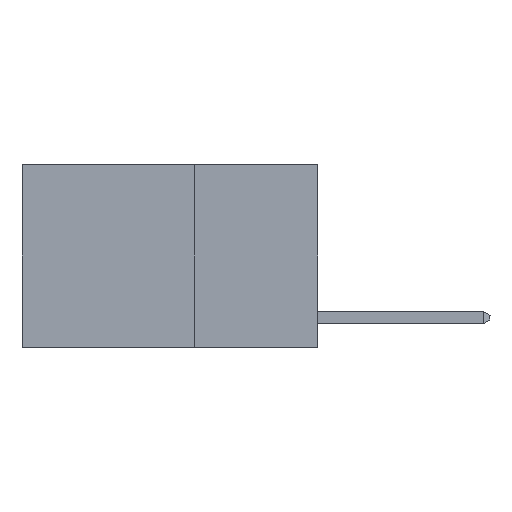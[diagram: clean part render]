
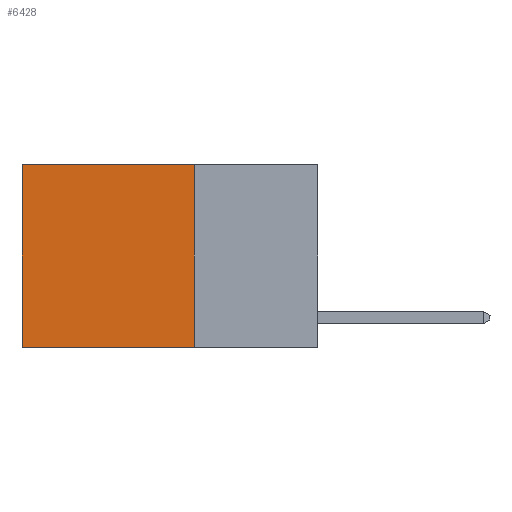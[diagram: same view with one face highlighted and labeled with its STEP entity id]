
A CAD part, left-side view. The second image highlights one B-rep face of the part: STEP entity #6428.
In plain terms, the highlighted planar face has unit normal (-1, 0, 0).
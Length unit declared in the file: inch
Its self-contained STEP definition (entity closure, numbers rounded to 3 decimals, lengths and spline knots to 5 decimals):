
#82 = LINE ( 'NONE', #4856, #4059 ) ;
#252 = ORIENTED_EDGE ( 'NONE', *, *, #3292, .T. ) ;
#407 = EDGE_CURVE ( 'NONE', #6650, #4526, #2956, .T. ) ;
#755 = CARTESIAN_POINT ( 'NONE',  ( 0.2625, 0.25, 0. ) ) ;
#857 = EDGE_CURVE ( 'NONE', #6430, #4526, #6708, .T. ) ;
#1067 = VECTOR ( 'NONE', #3696, 39.37008 ) ;
#1344 = CARTESIAN_POINT ( 'NONE',  ( 0.2625, 0.6, 0. ) ) ;
#2021 = DIRECTION ( 'NONE',  ( 0., 1., 0. ) ) ;
#2533 = ORIENTED_EDGE ( 'NONE', *, *, #6698, .F. ) ;
#2956 = LINE ( 'NONE', #3728, #8029 ) ;
#3292 = EDGE_CURVE ( 'NONE', #7259, #6650, #82, .T. ) ;
#3528 = CARTESIAN_POINT ( 'NONE',  ( 0.2625, 0.25, -0.37 ) ) ;
#3675 = CARTESIAN_POINT ( 'NONE',  ( 0.2625, 0.6, -0.37 ) ) ;
#3696 = DIRECTION ( 'NONE',  ( 0., 0., -1. ) ) ;
#3728 = CARTESIAN_POINT ( 'NONE',  ( 0.2625, 0.6, 0. ) ) ;
#4059 = VECTOR ( 'NONE', #2021, 39.37008 ) ;
#4200 = FACE_OUTER_BOUND ( 'NONE', #6991, .T. ) ;
#4526 = VERTEX_POINT ( 'NONE', #3675 ) ;
#4856 = CARTESIAN_POINT ( 'NONE',  ( 0.2625, 0.25, 0. ) ) ;
#5106 = DIRECTION ( 'NONE',  ( 0., 1., 0. ) ) ;
#5764 = CARTESIAN_POINT ( 'NONE',  ( 0.2625, 0.25, 0. ) ) ;
#6214 = ORIENTED_EDGE ( 'NONE', *, *, #407, .T. ) ;
#6428 = ADVANCED_FACE ( 'NONE', ( #4200 ), #8987, .F. ) ;
#6430 = VERTEX_POINT ( 'NONE', #3528 ) ;
#6650 = VERTEX_POINT ( 'NONE', #1344 ) ;
#6698 = EDGE_CURVE ( 'NONE', #7259, #6430, #7147, .T. ) ;
#6708 = LINE ( 'NONE', #8795, #7569 ) ;
#6877 = AXIS2_PLACEMENT_3D ( 'NONE', #755, #7707, #7754 ) ;
#6991 = EDGE_LOOP ( 'NONE', ( #6214, #8253, #2533, #252 ) ) ;
#7147 = LINE ( 'NONE', #5764, #1067 ) ;
#7181 = DIRECTION ( 'NONE',  ( 0., 0., -1. ) ) ;
#7259 = VERTEX_POINT ( 'NONE', #8933 ) ;
#7569 = VECTOR ( 'NONE', #5106, 39.37008 ) ;
#7707 = DIRECTION ( 'NONE',  ( 1., 0., 0. ) ) ;
#7754 = DIRECTION ( 'NONE',  ( 0., 0., -1. ) ) ;
#8029 = VECTOR ( 'NONE', #7181, 39.37008 ) ;
#8253 = ORIENTED_EDGE ( 'NONE', *, *, #857, .F. ) ;
#8795 = CARTESIAN_POINT ( 'NONE',  ( 0.2625, 0.25, -0.37 ) ) ;
#8933 = CARTESIAN_POINT ( 'NONE',  ( 0.2625, 0.25, 0. ) ) ;
#8987 = PLANE ( 'NONE',  #6877 ) ;
